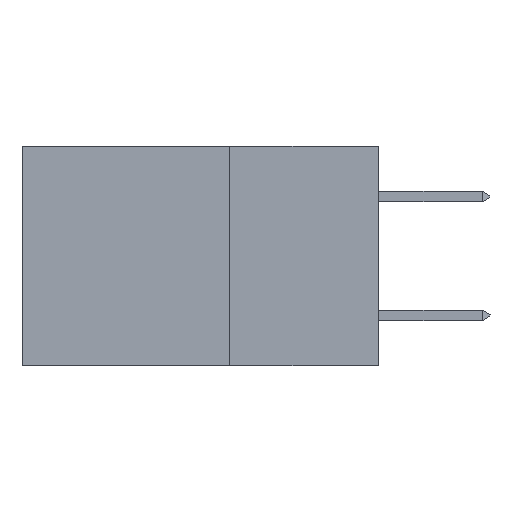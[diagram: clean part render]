
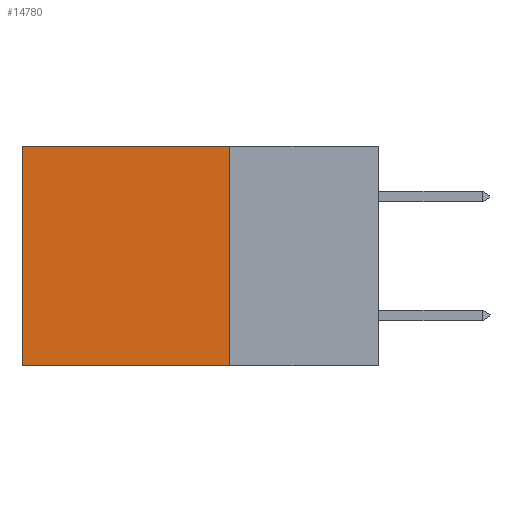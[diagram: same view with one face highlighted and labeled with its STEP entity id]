
A CAD part, left-side view. The second image highlights one B-rep face of the part: STEP entity #14780.
In plain terms, the highlighted planar face has unit normal (-1, 0, 0).
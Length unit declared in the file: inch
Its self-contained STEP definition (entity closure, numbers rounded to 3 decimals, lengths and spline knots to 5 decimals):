
#1079 = DIRECTION ( 'NONE',  ( 0., 0., -1. ) ) ;
#1380 = AXIS2_PLACEMENT_3D ( 'NONE', #18879, #19028, #4515 ) ;
#1587 = CARTESIAN_POINT ( 'NONE',  ( 0.298, 0.25, -0.37 ) ) ;
#1793 = LINE ( 'NONE', #5961, #16539 ) ;
#2747 = FACE_OUTER_BOUND ( 'NONE', #6597, .T. ) ;
#3358 = CARTESIAN_POINT ( 'NONE',  ( 0.298, 0.25, -0.37 ) ) ;
#4297 = LINE ( 'NONE', #13875, #16464 ) ;
#4515 = DIRECTION ( 'NONE',  ( 0., 0., -1. ) ) ;
#5013 = CARTESIAN_POINT ( 'NONE',  ( 0.298, 0.6, 0. ) ) ;
#5098 = VERTEX_POINT ( 'NONE', #3358 ) ;
#5332 = VECTOR ( 'NONE', #1079, 39.37008 ) ;
#5961 = CARTESIAN_POINT ( 'NONE',  ( 0.298, 0.6, 0. ) ) ;
#6597 = EDGE_LOOP ( 'NONE', ( #17699, #11824, #16810, #17589 ) ) ;
#8729 = VERTEX_POINT ( 'NONE', #5013 ) ;
#9105 = DIRECTION ( 'NONE',  ( 0., 1., 0. ) ) ;
#9272 = VERTEX_POINT ( 'NONE', #19088 ) ;
#9501 = VERTEX_POINT ( 'NONE', #18707 ) ;
#10221 = VECTOR ( 'NONE', #12937, 39.37008 ) ;
#10398 = EDGE_CURVE ( 'NONE', #9501, #5098, #12430, .T. ) ;
#11824 = ORIENTED_EDGE ( 'NONE', *, *, #15326, .F. ) ;
#12231 = PLANE ( 'NONE',  #1380 ) ;
#12430 = LINE ( 'NONE', #16967, #5332 ) ;
#12937 = DIRECTION ( 'NONE',  ( 0., 1., 0. ) ) ;
#13875 = CARTESIAN_POINT ( 'NONE',  ( 0.298, 0.25, 0. ) ) ;
#14780 = ADVANCED_FACE ( 'NONE', ( #2747 ), #12231, .F. ) ;
#15326 = EDGE_CURVE ( 'NONE', #5098, #9272, #16578, .T. ) ;
#16035 = EDGE_CURVE ( 'NONE', #8729, #9272, #1793, .T. ) ;
#16464 = VECTOR ( 'NONE', #9105, 39.37008 ) ;
#16539 = VECTOR ( 'NONE', #19121, 39.37008 ) ;
#16578 = LINE ( 'NONE', #1587, #10221 ) ;
#16810 = ORIENTED_EDGE ( 'NONE', *, *, #10398, .F. ) ;
#16967 = CARTESIAN_POINT ( 'NONE',  ( 0.298, 0.25, 0. ) ) ;
#17589 = ORIENTED_EDGE ( 'NONE', *, *, #18430, .T. ) ;
#17699 = ORIENTED_EDGE ( 'NONE', *, *, #16035, .T. ) ;
#18430 = EDGE_CURVE ( 'NONE', #9501, #8729, #4297, .T. ) ;
#18707 = CARTESIAN_POINT ( 'NONE',  ( 0.298, 0.25, 0. ) ) ;
#18879 = CARTESIAN_POINT ( 'NONE',  ( 0.298, 0.25, 0. ) ) ;
#19028 = DIRECTION ( 'NONE',  ( 1., 0., 0. ) ) ;
#19088 = CARTESIAN_POINT ( 'NONE',  ( 0.298, 0.6, -0.37 ) ) ;
#19121 = DIRECTION ( 'NONE',  ( 0., 0., -1. ) ) ;
